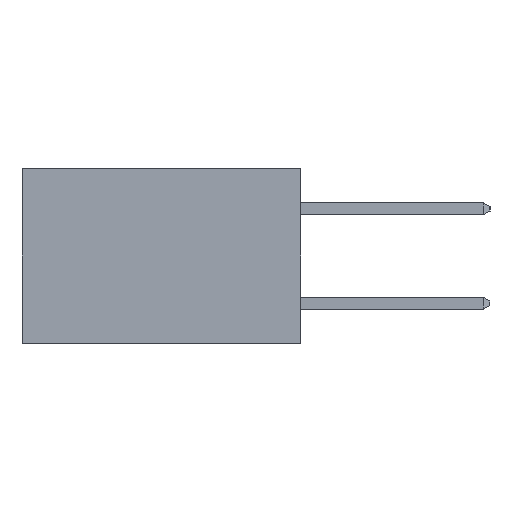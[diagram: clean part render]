
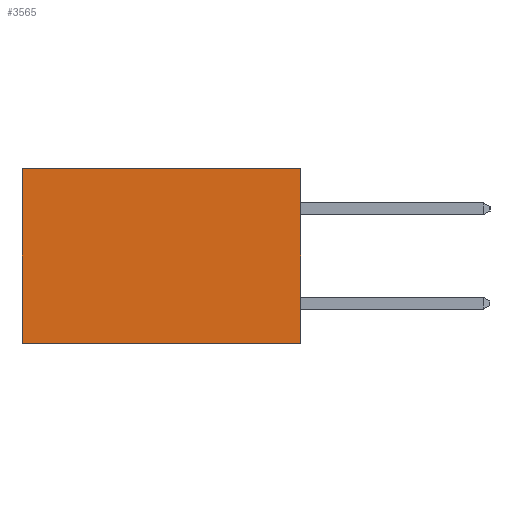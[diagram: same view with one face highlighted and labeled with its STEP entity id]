
A CAD part, left-side view. The second image highlights one B-rep face of the part: STEP entity #3565.
In plain terms, the highlighted planar face has unit normal (-1, 0, 0).
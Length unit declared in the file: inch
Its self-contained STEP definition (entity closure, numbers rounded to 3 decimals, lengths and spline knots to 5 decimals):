
#9 = CARTESIAN_POINT ( 'NONE',  ( 0.277, 0., -0.37 ) ) ;
#367 = CARTESIAN_POINT ( 'NONE',  ( 0.277, 0.59, -0.37 ) ) ;
#476 = EDGE_CURVE ( 'NONE', #9516, #15110, #5353, .T. ) ;
#675 = CARTESIAN_POINT ( 'NONE',  ( 0.277, 0.59, -0.37 ) ) ;
#1208 = VERTEX_POINT ( 'NONE', #11726 ) ;
#1797 = PLANE ( 'NONE',  #9326 ) ;
#1819 = VECTOR ( 'NONE', #8290, 39.37008 ) ;
#2074 = DIRECTION ( 'NONE',  ( 0., 0., -1. ) ) ;
#2327 = VECTOR ( 'NONE', #2074, 39.37008 ) ;
#3314 = EDGE_CURVE ( 'NONE', #1208, #9516, #7270, .T. ) ;
#3565 = ADVANCED_FACE ( 'NONE', ( #17139 ), #1797, .F. ) ;
#3720 = DIRECTION ( 'NONE',  ( 0., 0., -1. ) ) ;
#4030 = EDGE_LOOP ( 'NONE', ( #16700, #11905, #9739, #13424 ) ) ;
#4452 = DIRECTION ( 'NONE',  ( 1., 0., 0. ) ) ;
#5353 = LINE ( 'NONE', #6516, #15995 ) ;
#5682 = EDGE_CURVE ( 'NONE', #1208, #7212, #6437, .T. ) ;
#5689 = DIRECTION ( 'NONE',  ( 0., 1., 0. ) ) ;
#6437 = LINE ( 'NONE', #8197, #1819 ) ;
#6516 = CARTESIAN_POINT ( 'NONE',  ( 0.277, 0., -0.37 ) ) ;
#7212 = VERTEX_POINT ( 'NONE', #15895 ) ;
#7270 = LINE ( 'NONE', #12767, #17354 ) ;
#8197 = CARTESIAN_POINT ( 'NONE',  ( 0.277, 0., 0. ) ) ;
#8290 = DIRECTION ( 'NONE',  ( 0., 1., 0. ) ) ;
#9326 = AXIS2_PLACEMENT_3D ( 'NONE', #9, #4452, #3720 ) ;
#9516 = VERTEX_POINT ( 'NONE', #10993 ) ;
#9577 = DIRECTION ( 'NONE',  ( 0., 0., -1. ) ) ;
#9739 = ORIENTED_EDGE ( 'NONE', *, *, #3314, .F. ) ;
#9773 = LINE ( 'NONE', #675, #2327 ) ;
#9909 = EDGE_CURVE ( 'NONE', #7212, #15110, #9773, .T. ) ;
#10993 = CARTESIAN_POINT ( 'NONE',  ( 0.277, 0., -0.37 ) ) ;
#11726 = CARTESIAN_POINT ( 'NONE',  ( 0.277, 0., 0. ) ) ;
#11905 = ORIENTED_EDGE ( 'NONE', *, *, #476, .F. ) ;
#12767 = CARTESIAN_POINT ( 'NONE',  ( 0.277, 0., -0.37 ) ) ;
#13424 = ORIENTED_EDGE ( 'NONE', *, *, #5682, .T. ) ;
#15110 = VERTEX_POINT ( 'NONE', #367 ) ;
#15895 = CARTESIAN_POINT ( 'NONE',  ( 0.277, 0.59, 0. ) ) ;
#15995 = VECTOR ( 'NONE', #5689, 39.37008 ) ;
#16700 = ORIENTED_EDGE ( 'NONE', *, *, #9909, .T. ) ;
#17139 = FACE_OUTER_BOUND ( 'NONE', #4030, .T. ) ;
#17354 = VECTOR ( 'NONE', #9577, 39.37008 ) ;
